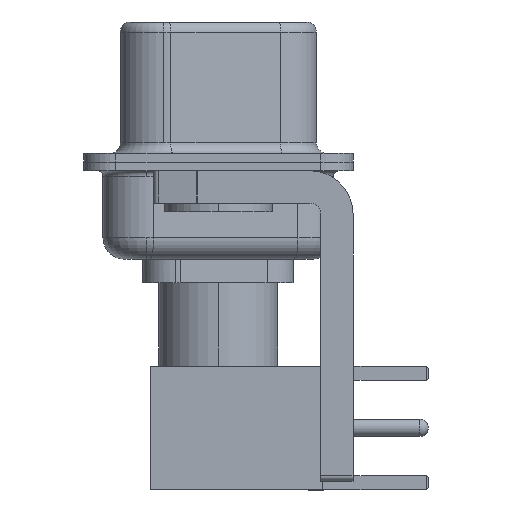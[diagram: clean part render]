
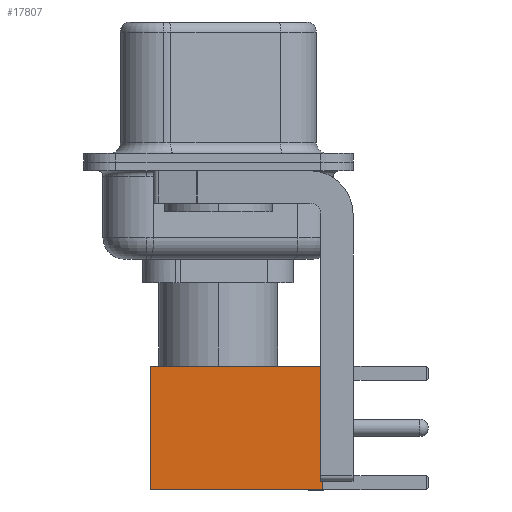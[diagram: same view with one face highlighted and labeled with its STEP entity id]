
A CAD part, left-side view. The second image highlights one B-rep face of the part: STEP entity #17807.
In plain terms, the highlighted face is planar.
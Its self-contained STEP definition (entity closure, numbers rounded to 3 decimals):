
#170 = LINE ( 'NONE', #11084, #16045 ) ;
#1111 = CARTESIAN_POINT ( 'NONE',  ( 2.875, 2.875, 8. ) ) ;
#1376 = EDGE_CURVE ( 'NONE', #12548, #18548, #18706, .T. ) ;
#2947 = VERTEX_POINT ( 'NONE', #1111 ) ;
#3360 = CARTESIAN_POINT ( 'NONE',  ( -2.875, 2.875, 8. ) ) ;
#4161 = LINE ( 'NONE', #9098, #15381 ) ;
#5015 = EDGE_CURVE ( 'NONE', #2947, #13379, #4161, .T. ) ;
#7646 = DIRECTION ( 'NONE',  ( -1., 0., 0. ) ) ;
#8626 = CARTESIAN_POINT ( 'NONE',  ( 2.875, 2.875, 0. ) ) ;
#9098 = CARTESIAN_POINT ( 'NONE',  ( 0., 2.875, 8. ) ) ;
#9328 = DIRECTION ( 'NONE',  ( 0., 0., -1. ) ) ;
#10010 = ORIENTED_EDGE ( 'NONE', *, *, #5015, .F. ) ;
#10173 = FACE_OUTER_BOUND ( 'NONE', #18511, .T. ) ;
#11084 = CARTESIAN_POINT ( 'NONE',  ( -2.875, 2.875, 0. ) ) ;
#11256 = VECTOR ( 'NONE', #15221, 1000. ) ;
#11619 = EDGE_CURVE ( 'NONE', #2947, #12548, #18034, .T. ) ;
#11664 = CARTESIAN_POINT ( 'NONE',  ( -2.875, 2.875, 0. ) ) ;
#11830 = PLANE ( 'NONE',  #18339 ) ;
#12210 = CARTESIAN_POINT ( 'NONE',  ( 0., 2.875, 0. ) ) ;
#12284 = ORIENTED_EDGE ( 'NONE', *, *, #19078, .F. ) ;
#12548 = VERTEX_POINT ( 'NONE', #13496 ) ;
#13369 = DIRECTION ( 'NONE',  ( 0., 1., 0. ) ) ;
#13379 = VERTEX_POINT ( 'NONE', #3360 ) ;
#13496 = CARTESIAN_POINT ( 'NONE',  ( 2.875, 2.875, 0. ) ) ;
#14815 = DIRECTION ( 'NONE',  ( 0., 0., 1. ) ) ;
#15221 = DIRECTION ( 'NONE',  ( 0., 0., -1. ) ) ;
#15381 = VECTOR ( 'NONE', #18705, 1000. ) ;
#15881 = CARTESIAN_POINT ( 'NONE',  ( 2.875, 2.875, 0. ) ) ;
#16045 = VECTOR ( 'NONE', #9328, 1000. ) ;
#16265 = ORIENTED_EDGE ( 'NONE', *, *, #1376, .T. ) ;
#17807 = ADVANCED_FACE ( 'NONE', ( #10173 ), #11830, .T. ) ;
#18034 = LINE ( 'NONE', #8626, #11256 ) ;
#18102 = ORIENTED_EDGE ( 'NONE', *, *, #11619, .T. ) ;
#18339 = AXIS2_PLACEMENT_3D ( 'NONE', #15881, #13369, #14815 ) ;
#18391 = VECTOR ( 'NONE', #7646, 1000. ) ;
#18511 = EDGE_LOOP ( 'NONE', ( #18102, #16265, #12284, #10010 ) ) ;
#18548 = VERTEX_POINT ( 'NONE', #11664 ) ;
#18705 = DIRECTION ( 'NONE',  ( -1., 0., 0. ) ) ;
#18706 = LINE ( 'NONE', #12210, #18391 ) ;
#19078 = EDGE_CURVE ( 'NONE', #13379, #18548, #170, .T. ) ;
